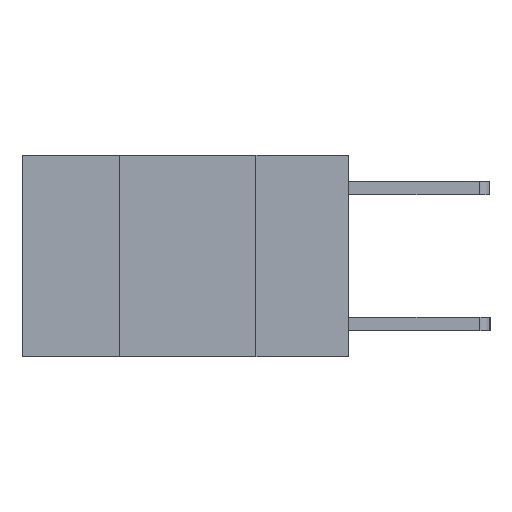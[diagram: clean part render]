
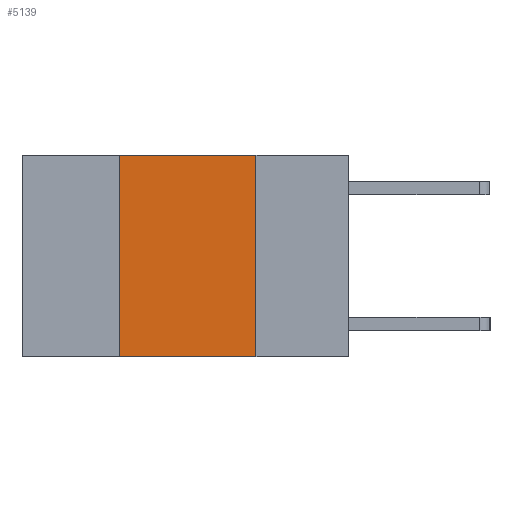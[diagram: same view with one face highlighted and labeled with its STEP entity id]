
A CAD part, left-side view. The second image highlights one B-rep face of the part: STEP entity #5139.
In plain terms, the highlighted planar face has unit normal (-1, 0, 0).
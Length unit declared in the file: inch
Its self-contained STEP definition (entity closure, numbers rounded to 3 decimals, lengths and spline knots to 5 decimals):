
#1147 = VERTEX_POINT ( 'NONE', #4242 ) ;
#1422 = CARTESIAN_POINT ( 'NONE',  ( 0., 0.42, -0.37 ) ) ;
#1717 = EDGE_CURVE ( 'NONE', #7726, #1147, #7822, .T. ) ;
#1856 = LINE ( 'NONE', #8396, #5686 ) ;
#1869 = ORIENTED_EDGE ( 'NONE', *, *, #4318, .F. ) ;
#1930 = CARTESIAN_POINT ( 'NONE',  ( 0., 0.6, 0. ) ) ;
#2346 = EDGE_LOOP ( 'NONE', ( #7521, #1869, #6625, #9752 ) ) ;
#2534 = VECTOR ( 'NONE', #9215, 39.37008 ) ;
#2636 = VECTOR ( 'NONE', #7522, 39.37008 ) ;
#2708 = DIRECTION ( 'NONE',  ( 0., 0., -1. ) ) ;
#2953 = AXIS2_PLACEMENT_3D ( 'NONE', #1930, #7232, #2708 ) ;
#2994 = CARTESIAN_POINT ( 'NONE',  ( 0., 0.17, 0. ) ) ;
#2996 = FACE_OUTER_BOUND ( 'NONE', #2346, .T. ) ;
#3142 = CARTESIAN_POINT ( 'NONE',  ( 0., 0.6, 0. ) ) ;
#3773 = VERTEX_POINT ( 'NONE', #9261 ) ;
#4242 = CARTESIAN_POINT ( 'NONE',  ( 0., 0.17, -0.37 ) ) ;
#4318 = EDGE_CURVE ( 'NONE', #3773, #7456, #8829, .T. ) ;
#5139 = ADVANCED_FACE ( 'NONE', ( #2996 ), #8737, .F. ) ;
#5456 = EDGE_CURVE ( 'NONE', #7456, #1147, #8922, .T. ) ;
#5686 = VECTOR ( 'NONE', #9156, 39.37008 ) ;
#5750 = CARTESIAN_POINT ( 'NONE',  ( 0., 0.17, 0. ) ) ;
#6625 = ORIENTED_EDGE ( 'NONE', *, *, #8281, .F. ) ;
#7232 = DIRECTION ( 'NONE',  ( 1., 0., 0. ) ) ;
#7456 = VERTEX_POINT ( 'NONE', #5750 ) ;
#7521 = ORIENTED_EDGE ( 'NONE', *, *, #5456, .F. ) ;
#7522 = DIRECTION ( 'NONE',  ( 0., 0., -1. ) ) ;
#7726 = VERTEX_POINT ( 'NONE', #1422 ) ;
#7822 = LINE ( 'NONE', #8868, #8059 ) ;
#8059 = VECTOR ( 'NONE', #8923, 39.37008 ) ;
#8281 = EDGE_CURVE ( 'NONE', #7726, #3773, #1856, .T. ) ;
#8396 = CARTESIAN_POINT ( 'NONE',  ( 0., 0.42, 0. ) ) ;
#8737 = PLANE ( 'NONE',  #2953 ) ;
#8829 = LINE ( 'NONE', #3142, #2534 ) ;
#8868 = CARTESIAN_POINT ( 'NONE',  ( 0., 0.6, -0.37 ) ) ;
#8922 = LINE ( 'NONE', #2994, #2636 ) ;
#8923 = DIRECTION ( 'NONE',  ( 0., -1., 0. ) ) ;
#9156 = DIRECTION ( 'NONE',  ( 0., 0., 1. ) ) ;
#9215 = DIRECTION ( 'NONE',  ( 0., -1., 0. ) ) ;
#9261 = CARTESIAN_POINT ( 'NONE',  ( 0., 0.42, 0. ) ) ;
#9752 = ORIENTED_EDGE ( 'NONE', *, *, #1717, .T. ) ;
